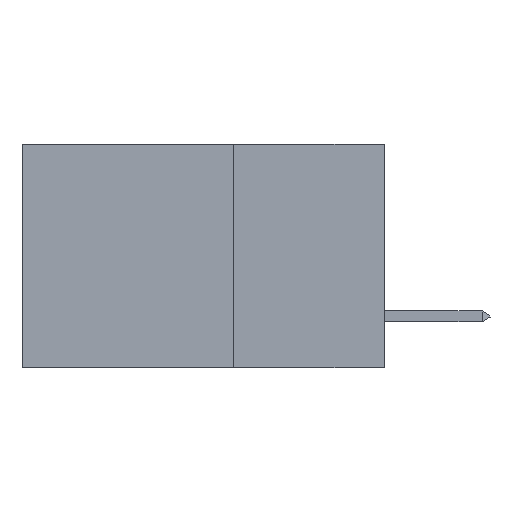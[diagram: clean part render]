
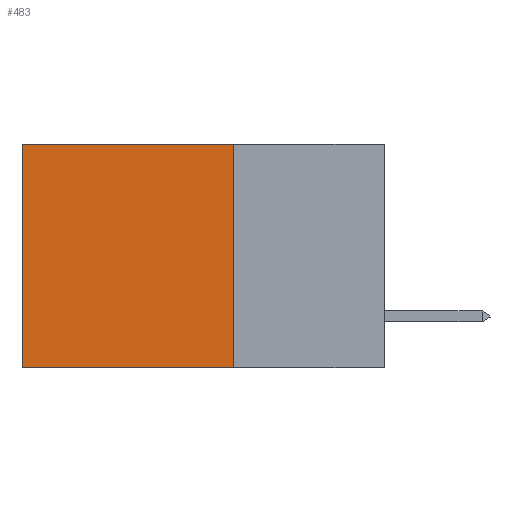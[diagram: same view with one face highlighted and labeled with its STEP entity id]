
A CAD part, left-side view. The second image highlights one B-rep face of the part: STEP entity #483.
In plain terms, the highlighted planar face has unit normal (-1, 0, 0).
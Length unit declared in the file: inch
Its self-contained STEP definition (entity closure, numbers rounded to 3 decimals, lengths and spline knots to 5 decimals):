
#483 = ADVANCED_FACE ( 'NONE', ( #1552 ), #12056, .F. ) ;
#1552 = FACE_OUTER_BOUND ( 'NONE', #11322, .T. ) ;
#2398 = CARTESIAN_POINT ( 'NONE',  ( 0.2875, 0.25, -0.37 ) ) ;
#3392 = ORIENTED_EDGE ( 'NONE', *, *, #6439, .T. ) ;
#3988 = LINE ( 'NONE', #17304, #25143 ) ;
#6439 = EDGE_CURVE ( 'NONE', #25222, #19486, #3988, .T. ) ;
#6571 = CARTESIAN_POINT ( 'NONE',  ( 0.2875, 0.25, 0. ) ) ;
#6815 = EDGE_CURVE ( 'NONE', #19486, #16310, #23044, .T. ) ;
#9916 = AXIS2_PLACEMENT_3D ( 'NONE', #13962, #10864, #32193 ) ;
#10864 = DIRECTION ( 'NONE',  ( 1., 0., 0. ) ) ;
#11322 = EDGE_LOOP ( 'NONE', ( #34519, #31779, #12653, #3392 ) ) ;
#12056 = PLANE ( 'NONE',  #9916 ) ;
#12622 = LINE ( 'NONE', #2398, #32488 ) ;
#12653 = ORIENTED_EDGE ( 'NONE', *, *, #26748, .F. ) ;
#13068 = DIRECTION ( 'NONE',  ( 0., 1., 0. ) ) ;
#13962 = CARTESIAN_POINT ( 'NONE',  ( 0.2875, 0.25, 0. ) ) ;
#16310 = VERTEX_POINT ( 'NONE', #28883 ) ;
#17304 = CARTESIAN_POINT ( 'NONE',  ( 0.2875, 0.25, 0. ) ) ;
#17938 = DIRECTION ( 'NONE',  ( 0., 0., -1. ) ) ;
#18313 = VERTEX_POINT ( 'NONE', #21893 ) ;
#19486 = VERTEX_POINT ( 'NONE', #23630 ) ;
#21847 = DIRECTION ( 'NONE',  ( 0., 1., 0. ) ) ;
#21893 = CARTESIAN_POINT ( 'NONE',  ( 0.2875, 0.25, -0.37 ) ) ;
#23044 = LINE ( 'NONE', #33981, #29284 ) ;
#23315 = DIRECTION ( 'NONE',  ( 0., 0., -1. ) ) ;
#23630 = CARTESIAN_POINT ( 'NONE',  ( 0.2875, 0.6, 0. ) ) ;
#25143 = VECTOR ( 'NONE', #13068, 39.37008 ) ;
#25222 = VERTEX_POINT ( 'NONE', #29907 ) ;
#26748 = EDGE_CURVE ( 'NONE', #25222, #18313, #34097, .T. ) ;
#28883 = CARTESIAN_POINT ( 'NONE',  ( 0.2875, 0.6, -0.37 ) ) ;
#29284 = VECTOR ( 'NONE', #17938, 39.37008 ) ;
#29907 = CARTESIAN_POINT ( 'NONE',  ( 0.2875, 0.25, 0. ) ) ;
#30172 = EDGE_CURVE ( 'NONE', #18313, #16310, #12622, .T. ) ;
#31779 = ORIENTED_EDGE ( 'NONE', *, *, #30172, .F. ) ;
#32193 = DIRECTION ( 'NONE',  ( 0., 0., -1. ) ) ;
#32446 = VECTOR ( 'NONE', #23315, 39.37008 ) ;
#32488 = VECTOR ( 'NONE', #21847, 39.37008 ) ;
#33981 = CARTESIAN_POINT ( 'NONE',  ( 0.2875, 0.6, 0. ) ) ;
#34097 = LINE ( 'NONE', #6571, #32446 ) ;
#34519 = ORIENTED_EDGE ( 'NONE', *, *, #6815, .T. ) ;
